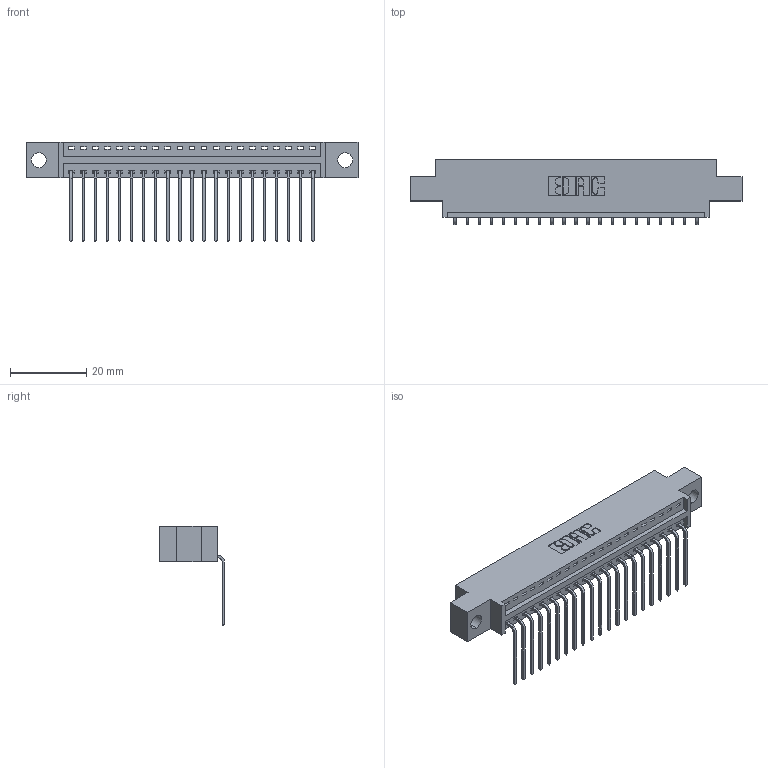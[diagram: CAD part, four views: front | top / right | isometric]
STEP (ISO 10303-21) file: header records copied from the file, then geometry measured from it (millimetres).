
FILE_DESCRIPTION (( 'STEP AP203' ), '1' );
FILE_NAME ('346-021-559-604.STEP', '2022-05-05T18:46:36', ( '' ), ( '' ), 'SwSTEP 2.0', 'SolidWorks 2020', '' );
FILE_SCHEMA (( 'CONFIG_CONTROL_DESIGN' ));
Length unit declared in the file: inch
Products named in the file (3): 346-021-559-604; 345-292-001_558 559 Tail - 1; 346 Part_0.170 Offset - 0.156 Dia-TH
Assembly tree (22 placements, depth 2):
  346-021-559-604
    346 Part_0.170 Offset - 0.156 Dia-TH
    345-292-001_558 559 Tail - 1  x21
Bounding box: 87.25 x 17.08 x 26.16 mm (x, y, z)
Volume: 8016.4 mm3; surface area: 10207.8 mm2
Topology: 22 solids, 22 shells, 1400 faces, 4199 edges, 2770 vertices
Faces by surface type: plane 976, cylinder 424
Entity records: 16495 total; most frequent: CARTESIAN_POINT 2845, ORIENTED_EDGE 2798, DIRECTION 2533, EDGE_CURVE 1399, VECTOR 1183, LINE 1183, VERTEX_POINT 930, AXIS2_PLACEMENT_3D 675
